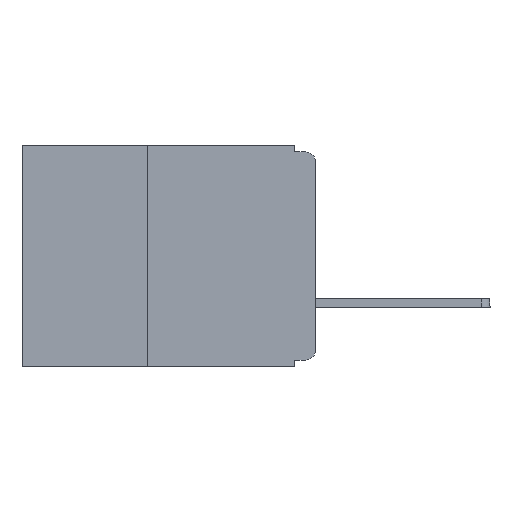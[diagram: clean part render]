
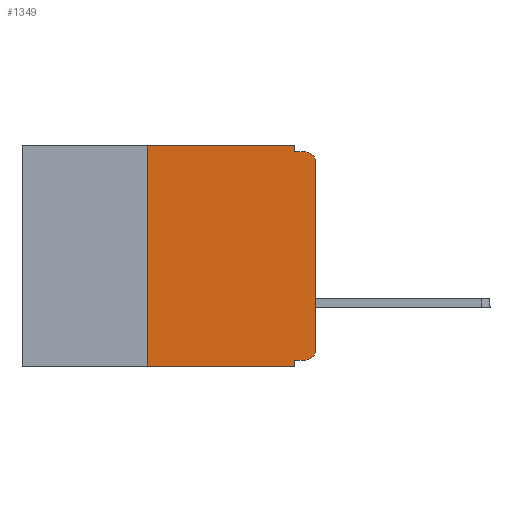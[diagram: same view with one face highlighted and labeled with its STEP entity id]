
A CAD part, left-side view. The second image highlights one B-rep face of the part: STEP entity #1349.
In plain terms, the highlighted planar face has unit normal (-1, 0, 0).
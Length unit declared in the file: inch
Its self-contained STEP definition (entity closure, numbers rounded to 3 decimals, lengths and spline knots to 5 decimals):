
#47 = EDGE_CURVE ( 'NONE', #9924, #7538, #10269, .T. ) ;
#289 = ORIENTED_EDGE ( 'NONE', *, *, #19483, .F. ) ;
#757 = AXIS2_PLACEMENT_3D ( 'NONE', #19767, #7482, #21857 ) ;
#965 = VECTOR ( 'NONE', #23983, 39.37008 ) ;
#1349 = ADVANCED_FACE ( 'NONE', ( #11606 ), #3792, .F. ) ;
#1469 = ORIENTED_EDGE ( 'NONE', *, *, #21818, .F. ) ;
#1588 = CARTESIAN_POINT ( 'NONE',  ( 0., 0.437, 0. ) ) ;
#2211 = LINE ( 'NONE', #3664, #11981 ) ;
#2260 = DIRECTION ( 'NONE',  ( 0., 1., 0. ) ) ;
#2733 = LINE ( 'NONE', #18162, #23937 ) ;
#2739 = ORIENTED_EDGE ( 'NONE', *, *, #11029, .F. ) ;
#3554 = CARTESIAN_POINT ( 'NONE',  ( 0., 0.031, -0.01 ) ) ;
#3556 = VECTOR ( 'NONE', #2260, 39.37008 ) ;
#3664 = CARTESIAN_POINT ( 'NONE',  ( 0., 0.031, -0.33 ) ) ;
#3792 = PLANE ( 'NONE',  #25294 ) ;
#4359 = CARTESIAN_POINT ( 'NONE',  ( 0., 0., -0.32 ) ) ;
#4476 = CARTESIAN_POINT ( 'NONE',  ( 0., 0., -0.01 ) ) ;
#4554 = CARTESIAN_POINT ( 'NONE',  ( 0., 0.015, -0.01 ) ) ;
#4581 = DIRECTION ( 'NONE',  ( 0., 0., 1. ) ) ;
#4669 = ORIENTED_EDGE ( 'NONE', *, *, #47, .T. ) ;
#4727 = VECTOR ( 'NONE', #4581, 39.37008 ) ;
#5425 = ORIENTED_EDGE ( 'NONE', *, *, #21351, .T. ) ;
#5808 = ORIENTED_EDGE ( 'NONE', *, *, #25544, .F. ) ;
#5843 = DIRECTION ( 'NONE',  ( 0., 0., -1. ) ) ;
#6058 = VERTEX_POINT ( 'NONE', #23675 ) ;
#6962 = VERTEX_POINT ( 'NONE', #22841 ) ;
#7077 = VERTEX_POINT ( 'NONE', #19150 ) ;
#7203 = EDGE_CURVE ( 'NONE', #20363, #10109, #17715, .T. ) ;
#7223 = CARTESIAN_POINT ( 'NONE',  ( 0., 0., 0. ) ) ;
#7294 = VERTEX_POINT ( 'NONE', #19866 ) ;
#7482 = DIRECTION ( 'NONE',  ( -1., 0., 0. ) ) ;
#7538 = VERTEX_POINT ( 'NONE', #12866 ) ;
#7593 = CARTESIAN_POINT ( 'NONE',  ( 0., 0.437, -0.33 ) ) ;
#7963 = DIRECTION ( 'NONE',  ( 0., 0., 1. ) ) ;
#8411 = DIRECTION ( 'NONE',  ( -1., 0., 0. ) ) ;
#9466 = AXIS2_PLACEMENT_3D ( 'NONE', #20682, #8411, #22723 ) ;
#9924 = VERTEX_POINT ( 'NONE', #18834 ) ;
#10109 = VERTEX_POINT ( 'NONE', #25532 ) ;
#10269 = LINE ( 'NONE', #7223, #4727 ) ;
#10948 = CIRCLE ( 'NONE', #757, 0.015 ) ;
#11029 = EDGE_CURVE ( 'NONE', #7294, #20363, #2733, .T. ) ;
#11606 = FACE_OUTER_BOUND ( 'NONE', #13602, .T. ) ;
#11649 = LINE ( 'NONE', #4476, #22464 ) ;
#11981 = VECTOR ( 'NONE', #13884, 39.37008 ) ;
#12628 = DIRECTION ( 'NONE',  ( 0., 0., -1. ) ) ;
#12691 = LINE ( 'NONE', #7593, #965 ) ;
#12866 = CARTESIAN_POINT ( 'NONE',  ( 0., 0., -0.025 ) ) ;
#13602 = EDGE_LOOP ( 'NONE', ( #4669, #5425, #15791, #289, #24470, #2739, #14421, #1469, #5808, #17106 ) ) ;
#13884 = DIRECTION ( 'NONE',  ( 0., 0., -1. ) ) ;
#14421 = ORIENTED_EDGE ( 'NONE', *, *, #19871, .T. ) ;
#14516 = LINE ( 'NONE', #4359, #3556 ) ;
#14845 = VERTEX_POINT ( 'NONE', #4554 ) ;
#15530 = LINE ( 'NONE', #16658, #20976 ) ;
#15791 = ORIENTED_EDGE ( 'NONE', *, *, #22052, .F. ) ;
#15804 = VECTOR ( 'NONE', #25763, 39.37008 ) ;
#16658 = CARTESIAN_POINT ( 'NONE',  ( 0., 0.031, 0. ) ) ;
#17106 = ORIENTED_EDGE ( 'NONE', *, *, #22943, .T. ) ;
#17715 = LINE ( 'NONE', #23714, #15804 ) ;
#17785 = CARTESIAN_POINT ( 'NONE',  ( 0., 0.25, 0. ) ) ;
#18144 = DIRECTION ( 'NONE',  ( 1., 0., 0. ) ) ;
#18162 = CARTESIAN_POINT ( 'NONE',  ( 0., 0.25, -0.33 ) ) ;
#18824 = DIRECTION ( 'NONE',  ( 0., -1., 0. ) ) ;
#18834 = CARTESIAN_POINT ( 'NONE',  ( 0., 0., -0.305 ) ) ;
#19150 = CARTESIAN_POINT ( 'NONE',  ( 0., 0.015, -0.32 ) ) ;
#19483 = EDGE_CURVE ( 'NONE', #10109, #25307, #15530, .T. ) ;
#19767 = CARTESIAN_POINT ( 'NONE',  ( 0., 0.015, -0.305 ) ) ;
#19866 = CARTESIAN_POINT ( 'NONE',  ( 0., 0.25, -0.33 ) ) ;
#19871 = EDGE_CURVE ( 'NONE', #7294, #6058, #12691, .T. ) ;
#20363 = VERTEX_POINT ( 'NONE', #17785 ) ;
#20682 = CARTESIAN_POINT ( 'NONE',  ( 0., 0.015, -0.025 ) ) ;
#20976 = VECTOR ( 'NONE', #12628, 39.37008 ) ;
#21351 = EDGE_CURVE ( 'NONE', #7538, #14845, #23443, .T. ) ;
#21818 = EDGE_CURVE ( 'NONE', #6962, #6058, #2211, .T. ) ;
#21857 = DIRECTION ( 'NONE',  ( 0., 0., -1. ) ) ;
#22052 = EDGE_CURVE ( 'NONE', #25307, #14845, #11649, .T. ) ;
#22464 = VECTOR ( 'NONE', #18824, 39.37008 ) ;
#22723 = DIRECTION ( 'NONE',  ( 0., 0., -1. ) ) ;
#22841 = CARTESIAN_POINT ( 'NONE',  ( 0., 0.031, -0.32 ) ) ;
#22943 = EDGE_CURVE ( 'NONE', #7077, #9924, #10948, .T. ) ;
#23443 = CIRCLE ( 'NONE', #9466, 0.015 ) ;
#23675 = CARTESIAN_POINT ( 'NONE',  ( 0., 0.031, -0.33 ) ) ;
#23714 = CARTESIAN_POINT ( 'NONE',  ( 0., 0.437, 0. ) ) ;
#23937 = VECTOR ( 'NONE', #7963, 39.37008 ) ;
#23983 = DIRECTION ( 'NONE',  ( 0., -1., 0. ) ) ;
#24470 = ORIENTED_EDGE ( 'NONE', *, *, #7203, .F. ) ;
#25294 = AXIS2_PLACEMENT_3D ( 'NONE', #1588, #18144, #5843 ) ;
#25307 = VERTEX_POINT ( 'NONE', #3554 ) ;
#25532 = CARTESIAN_POINT ( 'NONE',  ( 0., 0.031, 0. ) ) ;
#25544 = EDGE_CURVE ( 'NONE', #7077, #6962, #14516, .T. ) ;
#25763 = DIRECTION ( 'NONE',  ( 0., -1., 0. ) ) ;
